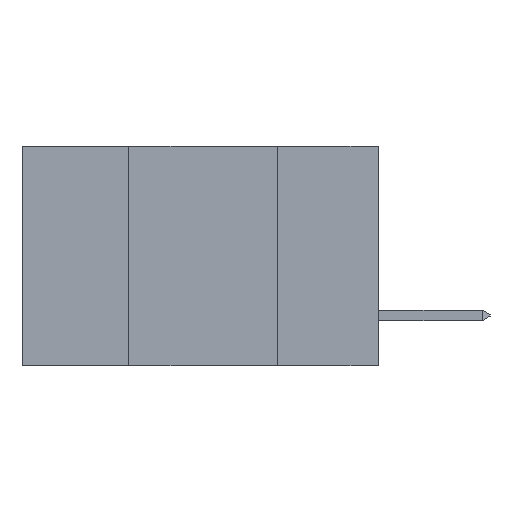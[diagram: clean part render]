
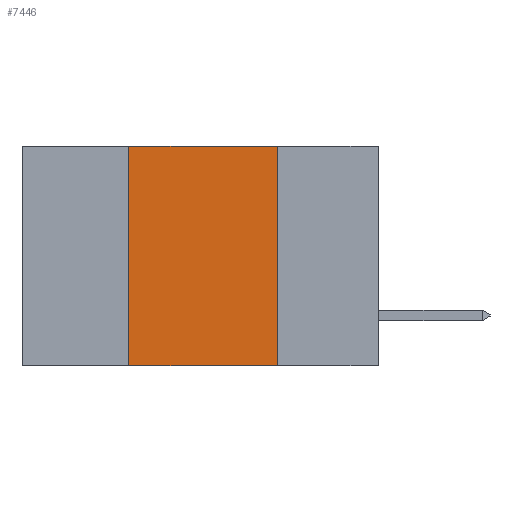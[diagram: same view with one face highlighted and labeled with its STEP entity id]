
A CAD part, left-side view. The second image highlights one B-rep face of the part: STEP entity #7446.
In plain terms, the highlighted planar face has unit normal (-1, 0, 0).
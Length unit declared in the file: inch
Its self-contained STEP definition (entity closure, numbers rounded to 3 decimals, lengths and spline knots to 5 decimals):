
#61 = DIRECTION ( 'NONE',  ( 0., 0., -1. ) ) ;
#253 = DIRECTION ( 'NONE',  ( 0., -1., 0. ) ) ;
#445 = CARTESIAN_POINT ( 'NONE',  ( 0., 0.42, -0.37 ) ) ;
#452 = VECTOR ( 'NONE', #253, 39.37008 ) ;
#946 = VECTOR ( 'NONE', #10710, 39.37008 ) ;
#962 = DIRECTION ( 'NONE',  ( 1., 0., 0. ) ) ;
#1148 = VERTEX_POINT ( 'NONE', #5262 ) ;
#1174 = VERTEX_POINT ( 'NONE', #1272 ) ;
#1222 = CARTESIAN_POINT ( 'NONE',  ( 0., 0.6, 0. ) ) ;
#1272 = CARTESIAN_POINT ( 'NONE',  ( 0., 0.17, -0.37 ) ) ;
#1600 = FACE_OUTER_BOUND ( 'NONE', #8940, .T. ) ;
#2477 = ORIENTED_EDGE ( 'NONE', *, *, #10418, .T. ) ;
#3962 = VERTEX_POINT ( 'NONE', #8930 ) ;
#4256 = EDGE_CURVE ( 'NONE', #3962, #1174, #9383, .T. ) ;
#5028 = CARTESIAN_POINT ( 'NONE',  ( 0., 0.42, -0.37 ) ) ;
#5136 = LINE ( 'NONE', #10619, #452 ) ;
#5262 = CARTESIAN_POINT ( 'NONE',  ( 0., 0.42, 0. ) ) ;
#5646 = EDGE_CURVE ( 'NONE', #11880, #1148, #5903, .T. ) ;
#5673 = CARTESIAN_POINT ( 'NONE',  ( 0., 0.17, -0.37 ) ) ;
#5903 = LINE ( 'NONE', #5028, #946 ) ;
#6569 = PLANE ( 'NONE',  #7432 ) ;
#7377 = VECTOR ( 'NONE', #8766, 39.37008 ) ;
#7432 = AXIS2_PLACEMENT_3D ( 'NONE', #12151, #962, #7512 ) ;
#7446 = ADVANCED_FACE ( 'NONE', ( #1600 ), #6569, .F. ) ;
#7512 = DIRECTION ( 'NONE',  ( 0., 0., -1. ) ) ;
#7580 = ORIENTED_EDGE ( 'NONE', *, *, #9563, .F. ) ;
#8478 = VECTOR ( 'NONE', #61, 39.37008 ) ;
#8766 = DIRECTION ( 'NONE',  ( 0., -1., 0. ) ) ;
#8930 = CARTESIAN_POINT ( 'NONE',  ( 0., 0.17, 0. ) ) ;
#8940 = EDGE_LOOP ( 'NONE', ( #9967, #7580, #11563, #2477 ) ) ;
#9383 = LINE ( 'NONE', #5673, #8478 ) ;
#9563 = EDGE_CURVE ( 'NONE', #1148, #3962, #9917, .T. ) ;
#9917 = LINE ( 'NONE', #1222, #7377 ) ;
#9967 = ORIENTED_EDGE ( 'NONE', *, *, #4256, .F. ) ;
#10418 = EDGE_CURVE ( 'NONE', #11880, #1174, #5136, .T. ) ;
#10619 = CARTESIAN_POINT ( 'NONE',  ( 0., 0.6, -0.37 ) ) ;
#10710 = DIRECTION ( 'NONE',  ( 0., 0., 1. ) ) ;
#11563 = ORIENTED_EDGE ( 'NONE', *, *, #5646, .F. ) ;
#11880 = VERTEX_POINT ( 'NONE', #445 ) ;
#12151 = CARTESIAN_POINT ( 'NONE',  ( 0., 0.6, 0. ) ) ;
